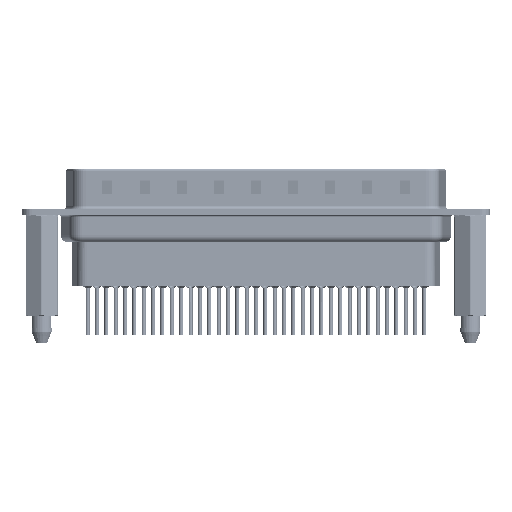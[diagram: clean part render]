
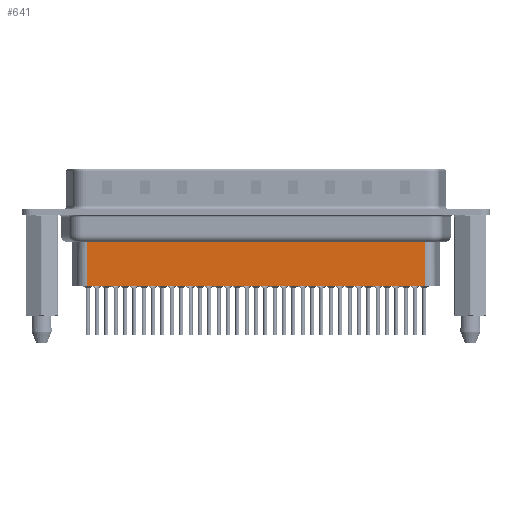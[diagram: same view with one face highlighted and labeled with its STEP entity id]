
A CAD part, front view. The second image highlights one B-rep face of the part: STEP entity #641.
In plain terms, the highlighted planar face has unit normal (0, -1, 0).
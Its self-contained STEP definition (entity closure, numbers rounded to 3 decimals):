
#641 = ADVANCED_FACE ( 'NONE', ( #25131 ), #2685, .T. ) ;
#1040 = CARTESIAN_POINT ( 'NONE',  ( 6.706, -3.5, -10.95 ) ) ;
#2186 = VERTEX_POINT ( 'NONE', #10795 ) ;
#2685 = PLANE ( 'NONE',  #25219 ) ;
#4544 = EDGE_LOOP ( 'NONE', ( #11755, #11995, #20009, #25061 ) ) ;
#4783 = VERTEX_POINT ( 'NONE', #5864 ) ;
#5864 = CARTESIAN_POINT ( 'NONE',  ( 56.794, -3.5, -10.95 ) ) ;
#6644 = DIRECTION ( 'NONE',  ( 0., 0., -1. ) ) ;
#6889 = EDGE_CURVE ( 'NONE', #7962, #4783, #16387, .T. ) ;
#7962 = VERTEX_POINT ( 'NONE', #30334 ) ;
#8048 = DIRECTION ( 'NONE',  ( 1., 0., 0. ) ) ;
#8663 = EDGE_CURVE ( 'NONE', #4783, #23512, #11042, .T. ) ;
#9056 = LINE ( 'NONE', #18971, #17020 ) ;
#10795 = CARTESIAN_POINT ( 'NONE',  ( 6.706, -3.5, -4.097 ) ) ;
#11042 = LINE ( 'NONE', #31232, #22309 ) ;
#11755 = ORIENTED_EDGE ( 'NONE', *, *, #6889, .F. ) ;
#11995 = ORIENTED_EDGE ( 'NONE', *, *, #12683, .T. ) ;
#12683 = EDGE_CURVE ( 'NONE', #7962, #2186, #18814, .T. ) ;
#13487 = DIRECTION ( 'NONE',  ( -1., 0., 0. ) ) ;
#16387 = LINE ( 'NONE', #28950, #26289 ) ;
#16540 = CARTESIAN_POINT ( 'NONE',  ( 6.459, -3.5, -4.097 ) ) ;
#17020 = VECTOR ( 'NONE', #19131, 1000. ) ;
#17828 = VECTOR ( 'NONE', #28780, 1000. ) ;
#18814 = LINE ( 'NONE', #16540, #17828 ) ;
#18971 = CARTESIAN_POINT ( 'NONE',  ( 6.706, -3.5, -3.1 ) ) ;
#19131 = DIRECTION ( 'NONE',  ( 0., 0., -1. ) ) ;
#20009 = ORIENTED_EDGE ( 'NONE', *, *, #21394, .T. ) ;
#21394 = EDGE_CURVE ( 'NONE', #2186, #23512, #9056, .T. ) ;
#22309 = VECTOR ( 'NONE', #13487, 1000. ) ;
#22688 = CARTESIAN_POINT ( 'NONE',  ( 6.706, -3.5, -3.1 ) ) ;
#23009 = DIRECTION ( 'NONE',  ( 0., -1., 0. ) ) ;
#23512 = VERTEX_POINT ( 'NONE', #1040 ) ;
#25061 = ORIENTED_EDGE ( 'NONE', *, *, #8663, .F. ) ;
#25131 = FACE_OUTER_BOUND ( 'NONE', #4544, .T. ) ;
#25219 = AXIS2_PLACEMENT_3D ( 'NONE', #22688, #23009, #8048 ) ;
#26289 = VECTOR ( 'NONE', #6644, 1000. ) ;
#28780 = DIRECTION ( 'NONE',  ( -1., 0., 0. ) ) ;
#28950 = CARTESIAN_POINT ( 'NONE',  ( 56.794, -3.5, -3.1 ) ) ;
#30334 = CARTESIAN_POINT ( 'NONE',  ( 56.794, -3.5, -4.097 ) ) ;
#31232 = CARTESIAN_POINT ( 'NONE',  ( 6.706, -3.5, -10.95 ) ) ;
